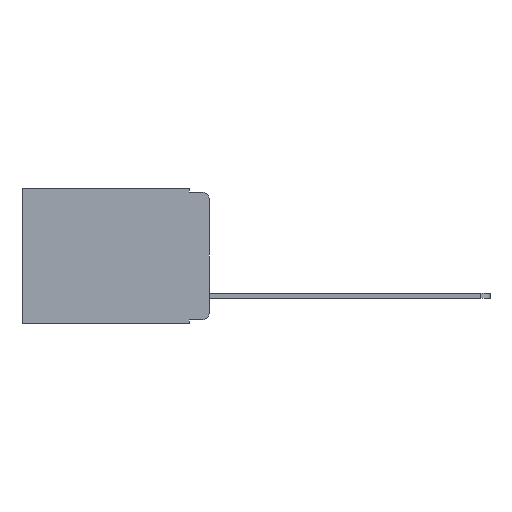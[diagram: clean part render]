
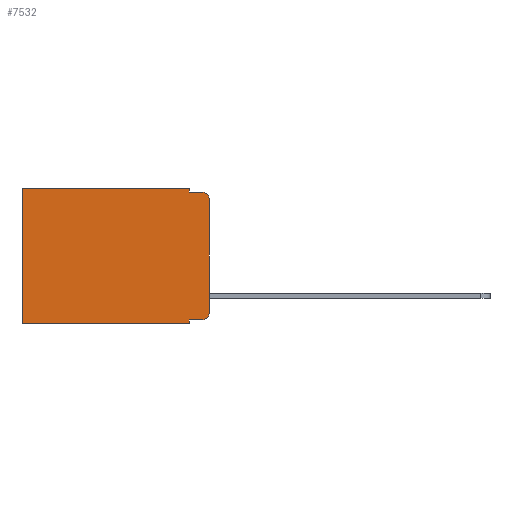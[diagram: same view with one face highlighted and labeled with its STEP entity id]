
A CAD part, left-side view. The second image highlights one B-rep face of the part: STEP entity #7532.
In plain terms, the highlighted planar face has unit normal (-1, 0, 0).
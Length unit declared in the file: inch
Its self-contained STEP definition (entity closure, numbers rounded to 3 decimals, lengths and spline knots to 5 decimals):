
#717 = VECTOR ( 'NONE', #8419, 39.37008 ) ;
#761 = VERTEX_POINT ( 'NONE', #12183 ) ;
#1061 = VERTEX_POINT ( 'NONE', #9884 ) ;
#1156 = CARTESIAN_POINT ( 'NONE',  ( 0.298, 0.473, -0.343 ) ) ;
#1218 = CARTESIAN_POINT ( 'NONE',  ( 0.298, 0.051, -0.01 ) ) ;
#1221 = CARTESIAN_POINT ( 'NONE',  ( 0.298, 0., -0.03 ) ) ;
#1309 = DIRECTION ( 'NONE',  ( 0., -1., 0. ) ) ;
#1404 = FACE_OUTER_BOUND ( 'NONE', #1857, .T. ) ;
#1439 = CARTESIAN_POINT ( 'NONE',  ( 0.298, 0., 0. ) ) ;
#1464 = EDGE_CURVE ( 'NONE', #6976, #10409, #12043, .T. ) ;
#1466 = VECTOR ( 'NONE', #1309, 39.37008 ) ;
#1646 = LINE ( 'NONE', #1439, #4866 ) ;
#1691 = CARTESIAN_POINT ( 'NONE',  ( 0.298, 0.02, -0.313 ) ) ;
#1857 = EDGE_LOOP ( 'NONE', ( #5347, #16124, #13133, #6614, #7036, #10477, #7448, #14378, #10887, #7866 ) ) ;
#1984 = CARTESIAN_POINT ( 'NONE',  ( 0.298, 0., -0.313 ) ) ;
#2151 = EDGE_CURVE ( 'NONE', #3671, #9455, #11400, .T. ) ;
#2157 = CARTESIAN_POINT ( 'NONE',  ( 0.298, 0.051, 0. ) ) ;
#2215 = DIRECTION ( 'NONE',  ( 0., 0., -1. ) ) ;
#2810 = VECTOR ( 'NONE', #9911, 39.37008 ) ;
#3044 = DIRECTION ( 'NONE',  ( 0., 0., -1. ) ) ;
#3074 = DIRECTION ( 'NONE',  ( 0., 0., -1. ) ) ;
#3467 = LINE ( 'NONE', #14724, #16996 ) ;
#3508 = CARTESIAN_POINT ( 'NONE',  ( 0.298, 0.051, 0. ) ) ;
#3671 = VERTEX_POINT ( 'NONE', #8693 ) ;
#4164 = CARTESIAN_POINT ( 'NONE',  ( 0.298, 0.051, -0.343 ) ) ;
#4734 = VECTOR ( 'NONE', #3044, 39.37008 ) ;
#4813 = EDGE_CURVE ( 'NONE', #761, #1061, #8687, .T. ) ;
#4866 = VECTOR ( 'NONE', #9563, 39.37008 ) ;
#5228 = PLANE ( 'NONE',  #13398 ) ;
#5347 = ORIENTED_EDGE ( 'NONE', *, *, #12297, .F. ) ;
#5555 = VECTOR ( 'NONE', #2215, 39.37008 ) ;
#5652 = VERTEX_POINT ( 'NONE', #1984 ) ;
#5710 = EDGE_CURVE ( 'NONE', #1061, #10409, #15149, .T. ) ;
#6614 = ORIENTED_EDGE ( 'NONE', *, *, #4813, .F. ) ;
#6926 = CARTESIAN_POINT ( 'NONE',  ( 0.298, 0., 0. ) ) ;
#6976 = VERTEX_POINT ( 'NONE', #1221 ) ;
#7036 = ORIENTED_EDGE ( 'NONE', *, *, #13511, .T. ) ;
#7081 = VERTEX_POINT ( 'NONE', #4164 ) ;
#7448 = ORIENTED_EDGE ( 'NONE', *, *, #15006, .F. ) ;
#7532 = ADVANCED_FACE ( 'NONE', ( #1404 ), #5228, .F. ) ;
#7866 = ORIENTED_EDGE ( 'NONE', *, *, #11754, .T. ) ;
#7922 = CARTESIAN_POINT ( 'NONE',  ( 0.298, 0., 0. ) ) ;
#8419 = DIRECTION ( 'NONE',  ( 0., 0., -1. ) ) ;
#8687 = LINE ( 'NONE', #3508, #4734 ) ;
#8693 = CARTESIAN_POINT ( 'NONE',  ( 0.298, 0.473, 0. ) ) ;
#8916 = AXIS2_PLACEMENT_3D ( 'NONE', #11946, #11742, #9843 ) ;
#9088 = LINE ( 'NONE', #2157, #5555 ) ;
#9223 = DIRECTION ( 'NONE',  ( 0., 0., -1. ) ) ;
#9455 = VERTEX_POINT ( 'NONE', #1156 ) ;
#9563 = DIRECTION ( 'NONE',  ( 0., 1., 0. ) ) ;
#9692 = CIRCLE ( 'NONE', #16650, 0.02 ) ;
#9801 = CARTESIAN_POINT ( 'NONE',  ( 0.298, 0.051, -0.333 ) ) ;
#9843 = DIRECTION ( 'NONE',  ( 0., 0., -1. ) ) ;
#9884 = CARTESIAN_POINT ( 'NONE',  ( 0.298, 0.051, -0.01 ) ) ;
#9911 = DIRECTION ( 'NONE',  ( 0., 1., 0. ) ) ;
#9923 = CARTESIAN_POINT ( 'NONE',  ( 0.298, 0.02, -0.01 ) ) ;
#10207 = EDGE_CURVE ( 'NONE', #14962, #16705, #3467, .T. ) ;
#10352 = CARTESIAN_POINT ( 'NONE',  ( 0.298, 0.473, 0. ) ) ;
#10409 = VERTEX_POINT ( 'NONE', #9923 ) ;
#10477 = ORIENTED_EDGE ( 'NONE', *, *, #2151, .T. ) ;
#10667 = VECTOR ( 'NONE', #14781, 39.37008 ) ;
#10887 = ORIENTED_EDGE ( 'NONE', *, *, #10207, .T. ) ;
#11027 = DIRECTION ( 'NONE',  ( -1., 0., 0. ) ) ;
#11400 = LINE ( 'NONE', #10352, #717 ) ;
#11742 = DIRECTION ( 'NONE',  ( -1., 0., 0. ) ) ;
#11754 = EDGE_CURVE ( 'NONE', #16705, #5652, #9692, .T. ) ;
#11946 = CARTESIAN_POINT ( 'NONE',  ( 0.298, 0.02, -0.03 ) ) ;
#11976 = EDGE_CURVE ( 'NONE', #14962, #7081, #9088, .T. ) ;
#12043 = CIRCLE ( 'NONE', #8916, 0.02 ) ;
#12183 = CARTESIAN_POINT ( 'NONE',  ( 0.298, 0.051, 0. ) ) ;
#12297 = EDGE_CURVE ( 'NONE', #6976, #5652, #14160, .T. ) ;
#12310 = CARTESIAN_POINT ( 'NONE',  ( 0.298, 0.02, -0.333 ) ) ;
#12531 = CARTESIAN_POINT ( 'NONE',  ( 0.298, 0., -0.343 ) ) ;
#13133 = ORIENTED_EDGE ( 'NONE', *, *, #5710, .F. ) ;
#13398 = AXIS2_PLACEMENT_3D ( 'NONE', #7922, #16948, #9223 ) ;
#13511 = EDGE_CURVE ( 'NONE', #761, #3671, #1646, .T. ) ;
#14160 = LINE ( 'NONE', #6926, #10667 ) ;
#14378 = ORIENTED_EDGE ( 'NONE', *, *, #11976, .F. ) ;
#14724 = CARTESIAN_POINT ( 'NONE',  ( 0.298, 0.051, -0.333 ) ) ;
#14781 = DIRECTION ( 'NONE',  ( 0., 0., -1. ) ) ;
#14962 = VERTEX_POINT ( 'NONE', #9801 ) ;
#15006 = EDGE_CURVE ( 'NONE', #7081, #9455, #15581, .T. ) ;
#15149 = LINE ( 'NONE', #1218, #1466 ) ;
#15581 = LINE ( 'NONE', #12531, #2810 ) ;
#15974 = DIRECTION ( 'NONE',  ( 0., -1., 0. ) ) ;
#16124 = ORIENTED_EDGE ( 'NONE', *, *, #1464, .T. ) ;
#16650 = AXIS2_PLACEMENT_3D ( 'NONE', #1691, #11027, #3074 ) ;
#16705 = VERTEX_POINT ( 'NONE', #12310 ) ;
#16948 = DIRECTION ( 'NONE',  ( 1., 0., 0. ) ) ;
#16996 = VECTOR ( 'NONE', #15974, 39.37008 ) ;
